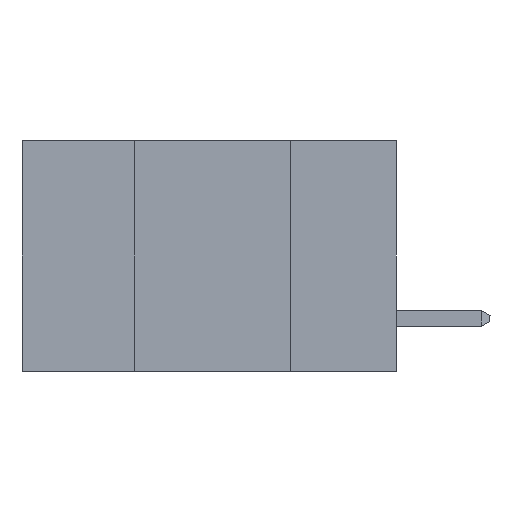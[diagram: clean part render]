
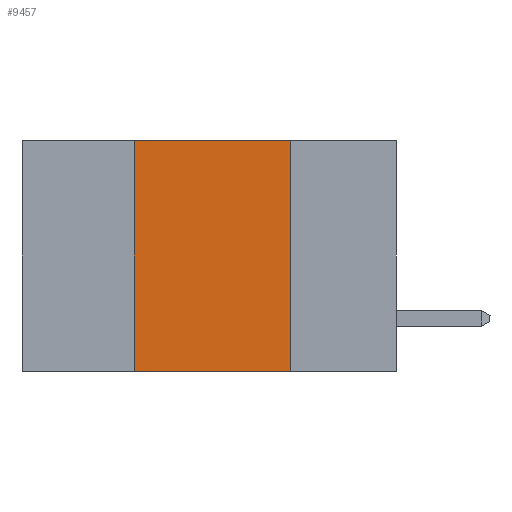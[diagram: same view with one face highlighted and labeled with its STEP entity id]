
A CAD part, left-side view. The second image highlights one B-rep face of the part: STEP entity #9457.
In plain terms, the highlighted planar face has unit normal (-1, 0, 0).
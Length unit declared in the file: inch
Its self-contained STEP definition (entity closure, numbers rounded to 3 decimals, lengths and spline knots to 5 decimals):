
#119 = AXIS2_PLACEMENT_3D ( 'NONE', #363, #5148, #6820 ) ;
#203 = LINE ( 'NONE', #7621, #4175 ) ;
#363 = CARTESIAN_POINT ( 'NONE',  ( 0., 0.6, 0. ) ) ;
#480 = CARTESIAN_POINT ( 'NONE',  ( 0., 0.17, -0.37 ) ) ;
#1069 = VERTEX_POINT ( 'NONE', #2455 ) ;
#1276 = EDGE_LOOP ( 'NONE', ( #3994, #7262, #1428, #3568 ) ) ;
#1428 = ORIENTED_EDGE ( 'NONE', *, *, #2176, .F. ) ;
#2146 = VERTEX_POINT ( 'NONE', #9322 ) ;
#2157 = LINE ( 'NONE', #4638, #2686 ) ;
#2176 = EDGE_CURVE ( 'NONE', #8906, #2146, #203, .T. ) ;
#2388 = DIRECTION ( 'NONE',  ( 0., 0., -1. ) ) ;
#2401 = DIRECTION ( 'NONE',  ( 0., -1., 0. ) ) ;
#2455 = CARTESIAN_POINT ( 'NONE',  ( 0., 0.17, 0. ) ) ;
#2579 = DIRECTION ( 'NONE',  ( 0., 0., 1. ) ) ;
#2686 = VECTOR ( 'NONE', #6234, 39.37008 ) ;
#2842 = FACE_OUTER_BOUND ( 'NONE', #1276, .T. ) ;
#3206 = VECTOR ( 'NONE', #2388, 39.37008 ) ;
#3568 = ORIENTED_EDGE ( 'NONE', *, *, #9758, .T. ) ;
#3994 = ORIENTED_EDGE ( 'NONE', *, *, #8570, .F. ) ;
#4175 = VECTOR ( 'NONE', #2579, 39.37008 ) ;
#4251 = VECTOR ( 'NONE', #2401, 39.37008 ) ;
#4638 = CARTESIAN_POINT ( 'NONE',  ( 0., 0.6, 0. ) ) ;
#5148 = DIRECTION ( 'NONE',  ( 1., 0., 0. ) ) ;
#6234 = DIRECTION ( 'NONE',  ( 0., -1., 0. ) ) ;
#6302 = VERTEX_POINT ( 'NONE', #480 ) ;
#6482 = LINE ( 'NONE', #9791, #4251 ) ;
#6564 = CARTESIAN_POINT ( 'NONE',  ( 0., 0.17, -0.37 ) ) ;
#6820 = DIRECTION ( 'NONE',  ( 0., 0., -1. ) ) ;
#7262 = ORIENTED_EDGE ( 'NONE', *, *, #8805, .F. ) ;
#7621 = CARTESIAN_POINT ( 'NONE',  ( 0., 0.42, -0.37 ) ) ;
#8066 = CARTESIAN_POINT ( 'NONE',  ( 0., 0.42, -0.37 ) ) ;
#8570 = EDGE_CURVE ( 'NONE', #1069, #6302, #9778, .T. ) ;
#8805 = EDGE_CURVE ( 'NONE', #2146, #1069, #2157, .T. ) ;
#8906 = VERTEX_POINT ( 'NONE', #8066 ) ;
#9322 = CARTESIAN_POINT ( 'NONE',  ( 0., 0.42, 0. ) ) ;
#9457 = ADVANCED_FACE ( 'NONE', ( #2842 ), #10160, .F. ) ;
#9758 = EDGE_CURVE ( 'NONE', #8906, #6302, #6482, .T. ) ;
#9778 = LINE ( 'NONE', #6564, #3206 ) ;
#9791 = CARTESIAN_POINT ( 'NONE',  ( 0., 0.6, -0.37 ) ) ;
#10160 = PLANE ( 'NONE',  #119 ) ;
